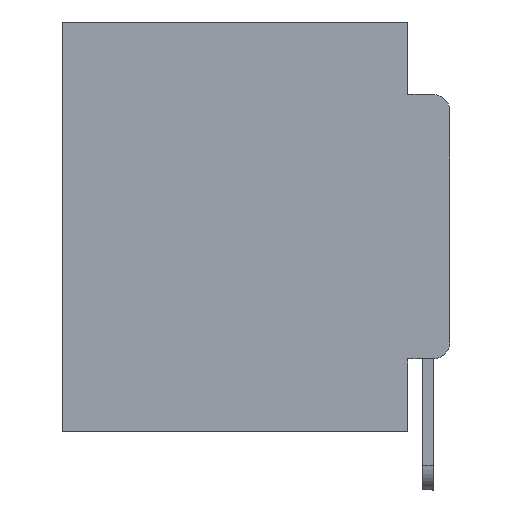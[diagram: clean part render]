
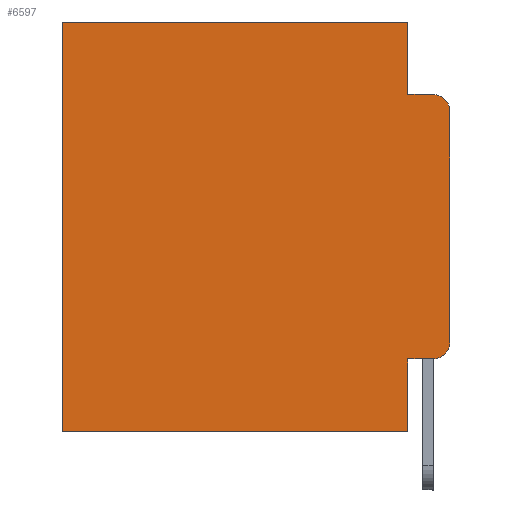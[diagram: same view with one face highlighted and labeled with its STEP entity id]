
A CAD part, left-side view. The second image highlights one B-rep face of the part: STEP entity #6597.
In plain terms, the highlighted planar face has unit normal (-1, 0, 0).
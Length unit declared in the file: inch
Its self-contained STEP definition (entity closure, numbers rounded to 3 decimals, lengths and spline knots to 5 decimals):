
#459 = CARTESIAN_POINT ( 'NONE',  ( 0.298, 0.02, -0.0885 ) ) ;
#515 = LINE ( 'NONE', #18630, #20367 ) ;
#545 = LINE ( 'NONE', #5160, #17623 ) ;
#796 = CARTESIAN_POINT ( 'NONE',  ( 0.298, 0.051, -0.0885 ) ) ;
#1096 = DIRECTION ( 'NONE',  ( 0., 0., -1. ) ) ;
#1351 = CIRCLE ( 'NONE', #16510, 0.02 ) ;
#1473 = ORIENTED_EDGE ( 'NONE', *, *, #17334, .F. ) ;
#1526 = CARTESIAN_POINT ( 'NONE',  ( 0.298, 0.473, 0. ) ) ;
#1551 = CARTESIAN_POINT ( 'NONE',  ( 0.298, 0.473, 0. ) ) ;
#2021 = DIRECTION ( 'NONE',  ( 0., 1., 0. ) ) ;
#2164 = VERTEX_POINT ( 'NONE', #1551 ) ;
#2166 = LINE ( 'NONE', #13444, #13972 ) ;
#2398 = EDGE_CURVE ( 'NONE', #20736, #26496, #1351, .T. ) ;
#2609 = PLANE ( 'NONE',  #5576 ) ;
#2739 = CARTESIAN_POINT ( 'NONE',  ( 0.298, 0.051, -0.0885 ) ) ;
#2892 = DIRECTION ( 'NONE',  ( 0., 0., -1. ) ) ;
#4522 = DIRECTION ( 'NONE',  ( 0., 1., 0. ) ) ;
#4926 = CARTESIAN_POINT ( 'NONE',  ( 0.298, 0.02, -0.4115 ) ) ;
#5160 = CARTESIAN_POINT ( 'NONE',  ( 0.298, 0.051, -0.4115 ) ) ;
#5302 = ORIENTED_EDGE ( 'NONE', *, *, #13477, .T. ) ;
#5462 = VECTOR ( 'NONE', #16091, 39.37008 ) ;
#5576 = AXIS2_PLACEMENT_3D ( 'NONE', #5978, #25755, #10144 ) ;
#5625 = ORIENTED_EDGE ( 'NONE', *, *, #14029, .F. ) ;
#5652 = LINE ( 'NONE', #16772, #16218 ) ;
#5978 = CARTESIAN_POINT ( 'NONE',  ( 0.298, 0., 0. ) ) ;
#6597 = ADVANCED_FACE ( 'NONE', ( #22937 ), #2609, .F. ) ;
#6800 = VECTOR ( 'NONE', #4522, 39.37008 ) ;
#7478 = CARTESIAN_POINT ( 'NONE',  ( 0.298, 0., -0.5 ) ) ;
#7589 = DIRECTION ( 'NONE',  ( 0., 0., -1. ) ) ;
#9105 = EDGE_CURVE ( 'NONE', #23920, #19160, #13737, .T. ) ;
#9363 = DIRECTION ( 'NONE',  ( -1., 0., 0. ) ) ;
#9930 = EDGE_CURVE ( 'NONE', #12520, #2164, #2166, .T. ) ;
#10144 = DIRECTION ( 'NONE',  ( 0., 0., -1. ) ) ;
#11433 = VERTEX_POINT ( 'NONE', #2739 ) ;
#11634 = DIRECTION ( 'NONE',  ( 0., 0., -1. ) ) ;
#12163 = ORIENTED_EDGE ( 'NONE', *, *, #14522, .F. ) ;
#12378 = CARTESIAN_POINT ( 'NONE',  ( 0.298, 0.051, -0.4115 ) ) ;
#12520 = VERTEX_POINT ( 'NONE', #25629 ) ;
#12765 = ORIENTED_EDGE ( 'NONE', *, *, #9930, .T. ) ;
#12768 = AXIS2_PLACEMENT_3D ( 'NONE', #16177, #9363, #24957 ) ;
#13444 = CARTESIAN_POINT ( 'NONE',  ( 0.298, 0., 0. ) ) ;
#13477 = EDGE_CURVE ( 'NONE', #24464, #23920, #545, .T. ) ;
#13737 = CIRCLE ( 'NONE', #12768, 0.02 ) ;
#13972 = VECTOR ( 'NONE', #2021, 39.37008 ) ;
#14029 = EDGE_CURVE ( 'NONE', #18825, #17095, #27797, .T. ) ;
#14174 = ORIENTED_EDGE ( 'NONE', *, *, #21821, .F. ) ;
#14522 = EDGE_CURVE ( 'NONE', #20736, #19160, #5652, .T. ) ;
#14998 = ORIENTED_EDGE ( 'NONE', *, *, #17444, .T. ) ;
#15645 = CARTESIAN_POINT ( 'NONE',  ( 0.298, 0.473, -0.5 ) ) ;
#16091 = DIRECTION ( 'NONE',  ( 0., -1., 0. ) ) ;
#16177 = CARTESIAN_POINT ( 'NONE',  ( 0.298, 0.02, -0.3915 ) ) ;
#16218 = VECTOR ( 'NONE', #7589, 39.37008 ) ;
#16510 = AXIS2_PLACEMENT_3D ( 'NONE', #17203, #21960, #2892 ) ;
#16772 = CARTESIAN_POINT ( 'NONE',  ( 0.298, 0., 0. ) ) ;
#17095 = VERTEX_POINT ( 'NONE', #15645 ) ;
#17203 = CARTESIAN_POINT ( 'NONE',  ( 0.298, 0.02, -0.1085 ) ) ;
#17334 = EDGE_CURVE ( 'NONE', #11433, #26496, #28106, .T. ) ;
#17444 = EDGE_CURVE ( 'NONE', #2164, #17095, #21863, .T. ) ;
#17623 = VECTOR ( 'NONE', #28154, 39.37008 ) ;
#17729 = ORIENTED_EDGE ( 'NONE', *, *, #21682, .F. ) ;
#18460 = VECTOR ( 'NONE', #11634, 39.37008 ) ;
#18630 = CARTESIAN_POINT ( 'NONE',  ( 0.298, 0.051, 0. ) ) ;
#18825 = VERTEX_POINT ( 'NONE', #24548 ) ;
#19160 = VERTEX_POINT ( 'NONE', #27214 ) ;
#20367 = VECTOR ( 'NONE', #27683, 39.37008 ) ;
#20736 = VERTEX_POINT ( 'NONE', #24082 ) ;
#21682 = EDGE_CURVE ( 'NONE', #24464, #18825, #24582, .T. ) ;
#21821 = EDGE_CURVE ( 'NONE', #12520, #11433, #515, .T. ) ;
#21863 = LINE ( 'NONE', #1526, #24900 ) ;
#21960 = DIRECTION ( 'NONE',  ( -1., 0., 0. ) ) ;
#22937 = FACE_OUTER_BOUND ( 'NONE', #29156, .T. ) ;
#23920 = VERTEX_POINT ( 'NONE', #4926 ) ;
#24082 = CARTESIAN_POINT ( 'NONE',  ( 0.298, 0., -0.1085 ) ) ;
#24464 = VERTEX_POINT ( 'NONE', #12378 ) ;
#24548 = CARTESIAN_POINT ( 'NONE',  ( 0.298, 0.051, -0.5 ) ) ;
#24582 = LINE ( 'NONE', #29019, #18460 ) ;
#24900 = VECTOR ( 'NONE', #1096, 39.37008 ) ;
#24957 = DIRECTION ( 'NONE',  ( 0., 0., -1. ) ) ;
#25555 = ORIENTED_EDGE ( 'NONE', *, *, #2398, .T. ) ;
#25629 = CARTESIAN_POINT ( 'NONE',  ( 0.298, 0.051, 0. ) ) ;
#25755 = DIRECTION ( 'NONE',  ( 1., 0., 0. ) ) ;
#26496 = VERTEX_POINT ( 'NONE', #459 ) ;
#27164 = ORIENTED_EDGE ( 'NONE', *, *, #9105, .T. ) ;
#27214 = CARTESIAN_POINT ( 'NONE',  ( 0.298, 0., -0.3915 ) ) ;
#27683 = DIRECTION ( 'NONE',  ( 0., 0., -1. ) ) ;
#27797 = LINE ( 'NONE', #7478, #6800 ) ;
#28106 = LINE ( 'NONE', #796, #5462 ) ;
#28154 = DIRECTION ( 'NONE',  ( 0., -1., 0. ) ) ;
#29019 = CARTESIAN_POINT ( 'NONE',  ( 0.298, 0.051, 0. ) ) ;
#29156 = EDGE_LOOP ( 'NONE', ( #12163, #25555, #1473, #14174, #12765, #14998, #5625, #17729, #5302, #27164 ) ) ;
